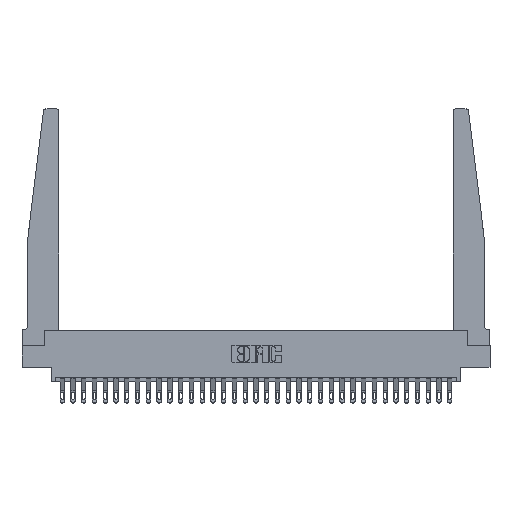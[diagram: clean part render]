
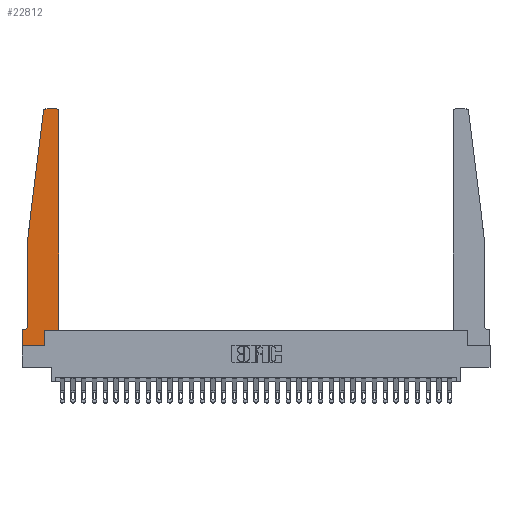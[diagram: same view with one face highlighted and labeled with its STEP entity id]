
A CAD part, top view. The second image highlights one B-rep face of the part: STEP entity #22812.
In plain terms, the highlighted planar face has unit normal (0, 0, 1).
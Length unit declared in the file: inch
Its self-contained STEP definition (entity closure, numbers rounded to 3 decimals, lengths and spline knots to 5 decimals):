
#106 = EDGE_CURVE ( 'NONE', #25178, #21801, #6517, .T. ) ;
#535 = EDGE_CURVE ( 'NONE', #23269, #25178, #2683, .T. ) ;
#1488 = EDGE_CURVE ( 'NONE', #19213, #11718, #28587, .T. ) ;
#2127 = CARTESIAN_POINT ( 'NONE',  ( 0.065, 0.2375, 0.37 ) ) ;
#2132 = VERTEX_POINT ( 'NONE', #7292 ) ;
#2136 = DIRECTION ( 'NONE',  ( 1., 0., 0. ) ) ;
#2334 = LINE ( 'NONE', #12359, #7658 ) ;
#2683 = LINE ( 'NONE', #5020, #24087 ) ;
#3017 = CARTESIAN_POINT ( 'NONE',  ( 0.2605, 0.18, 0.37 ) ) ;
#3242 = LINE ( 'NONE', #26306, #25599 ) ;
#3306 = CARTESIAN_POINT ( 'NONE',  ( 0.425, 0.18, 0.37 ) ) ;
#3314 = VERTEX_POINT ( 'NONE', #25134 ) ;
#3473 = LINE ( 'NONE', #21621, #29854 ) ;
#3608 = DIRECTION ( 'NONE',  ( 1., 0., 0. ) ) ;
#4772 = CARTESIAN_POINT ( 'NONE',  ( 0., 0., 0.37 ) ) ;
#5020 = CARTESIAN_POINT ( 'NONE',  ( 0.065, 1.25, 0.37 ) ) ;
#5546 = AXIS2_PLACEMENT_3D ( 'NONE', #10286, #24221, #7823 ) ;
#5682 = CARTESIAN_POINT ( 'NONE',  ( 0.065, 1.25, 0.37 ) ) ;
#5725 = ORIENTED_EDGE ( 'NONE', *, *, #16539, .T. ) ;
#6051 = DIRECTION ( 'NONE',  ( 0., 1., 0. ) ) ;
#6103 = DIRECTION ( 'NONE',  ( 1., 0., 0. ) ) ;
#6217 = ORIENTED_EDGE ( 'NONE', *, *, #535, .T. ) ;
#6342 = LINE ( 'NONE', #25376, #21973 ) ;
#6421 = DIRECTION ( 'NONE',  ( 0., 0., 1. ) ) ;
#6444 = ORIENTED_EDGE ( 'NONE', *, *, #16120, .T. ) ;
#6517 = CIRCLE ( 'NONE', #5546, 0.05 ) ;
#7292 = CARTESIAN_POINT ( 'NONE',  ( 0., 0., 0.37 ) ) ;
#7658 = VECTOR ( 'NONE', #21812, 39.37008 ) ;
#7823 = DIRECTION ( 'NONE',  ( -1., 0., 0. ) ) ;
#8012 = DIRECTION ( 'NONE',  ( 1., 0., 0. ) ) ;
#8994 = EDGE_CURVE ( 'NONE', #26713, #3314, #17209, .T. ) ;
#9644 = CARTESIAN_POINT ( 'NONE',  ( 0.425, 0.18, 0.37 ) ) ;
#9807 = ORIENTED_EDGE ( 'NONE', *, *, #15146, .T. ) ;
#9889 = DIRECTION ( 'NONE',  ( -1., 0., 0. ) ) ;
#10286 = CARTESIAN_POINT ( 'NONE',  ( 0.015, 0.2375, 0.37 ) ) ;
#10298 = LINE ( 'NONE', #5682, #20580 ) ;
#10486 = EDGE_CURVE ( 'NONE', #27199, #26713, #27411, .T. ) ;
#10804 = AXIS2_PLACEMENT_3D ( 'NONE', #27915, #6421, #22838 ) ;
#10860 = CARTESIAN_POINT ( 'NONE',  ( 0.395, 2.75, 0.37 ) ) ;
#11380 = LINE ( 'NONE', #4772, #18098 ) ;
#11718 = VERTEX_POINT ( 'NONE', #12896 ) ;
#11775 = DIRECTION ( 'NONE',  ( 0., 1., 0. ) ) ;
#11841 = ORIENTED_EDGE ( 'NONE', *, *, #13680, .T. ) ;
#12359 = CARTESIAN_POINT ( 'NONE',  ( 0., 0., 0.37 ) ) ;
#12484 = DIRECTION ( 'NONE',  ( 0., 0., 1. ) ) ;
#12896 = CARTESIAN_POINT ( 'NONE',  ( 0.24675, 2.72367, 0.37 ) ) ;
#13319 = CARTESIAN_POINT ( 'NONE',  ( 0.065, 1.25, 0.37 ) ) ;
#13458 = VECTOR ( 'NONE', #11775, 39.37008 ) ;
#13680 = EDGE_CURVE ( 'NONE', #11718, #23269, #10298, .T. ) ;
#14356 = CARTESIAN_POINT ( 'NONE',  ( 0.2605, 0., 0.37 ) ) ;
#15123 = ORIENTED_EDGE ( 'NONE', *, *, #8994, .T. ) ;
#15131 = CARTESIAN_POINT ( 'NONE',  ( 0., 0.1875, 0.37 ) ) ;
#15146 = EDGE_CURVE ( 'NONE', #15852, #19213, #3242, .T. ) ;
#15391 = ORIENTED_EDGE ( 'NONE', *, *, #18685, .T. ) ;
#15408 = CARTESIAN_POINT ( 'NONE',  ( 0.27653, 2.75, 0.37 ) ) ;
#15852 = VERTEX_POINT ( 'NONE', #10860 ) ;
#16120 = EDGE_CURVE ( 'NONE', #28943, #27199, #6342, .T. ) ;
#16298 = FACE_OUTER_BOUND ( 'NONE', #25149, .T. ) ;
#16539 = EDGE_CURVE ( 'NONE', #21801, #26189, #3473, .T. ) ;
#17039 = CARTESIAN_POINT ( 'NONE',  ( 0.015, 0.1875, 0.37 ) ) ;
#17209 = LINE ( 'NONE', #9644, #13458 ) ;
#17278 = CARTESIAN_POINT ( 'NONE',  ( 0.395, 2.72, 0.37 ) ) ;
#17915 = EDGE_CURVE ( 'NONE', #3314, #15852, #27969, .T. ) ;
#18098 = VECTOR ( 'NONE', #2136, 39.37008 ) ;
#18685 = EDGE_CURVE ( 'NONE', #26189, #2132, #2334, .T. ) ;
#18910 = DIRECTION ( 'NONE',  ( 0., -1., 0. ) ) ;
#19213 = VERTEX_POINT ( 'NONE', #15408 ) ;
#20157 = DIRECTION ( 'NONE',  ( -1., 0., 0. ) ) ;
#20580 = VECTOR ( 'NONE', #24856, 39.37008 ) ;
#20706 = EDGE_CURVE ( 'NONE', #2132, #28943, #11380, .T. ) ;
#20943 = ORIENTED_EDGE ( 'NONE', *, *, #20706, .T. ) ;
#21621 = CARTESIAN_POINT ( 'NONE',  ( 0.065, 0.1875, 0.37 ) ) ;
#21655 = ORIENTED_EDGE ( 'NONE', *, *, #106, .T. ) ;
#21801 = VERTEX_POINT ( 'NONE', #17039 ) ;
#21812 = DIRECTION ( 'NONE',  ( 0., -1., 0. ) ) ;
#21920 = CARTESIAN_POINT ( 'NONE',  ( 0.425, 0.18, 0.37 ) ) ;
#21973 = VECTOR ( 'NONE', #6051, 39.37008 ) ;
#22092 = DIRECTION ( 'NONE',  ( 0., 0., 1. ) ) ;
#22812 = ADVANCED_FACE ( 'NONE', ( #16298 ), #28072, .T. ) ;
#22838 = DIRECTION ( 'NONE',  ( 1., 0., 0. ) ) ;
#23269 = VERTEX_POINT ( 'NONE', #13319 ) ;
#24087 = VECTOR ( 'NONE', #18910, 39.37008 ) ;
#24124 = ORIENTED_EDGE ( 'NONE', *, *, #17915, .T. ) ;
#24221 = DIRECTION ( 'NONE',  ( 0., 0., -1. ) ) ;
#24658 = ORIENTED_EDGE ( 'NONE', *, *, #10486, .T. ) ;
#24856 = DIRECTION ( 'NONE',  ( -0.122, -0.992, 0. ) ) ;
#24993 = CARTESIAN_POINT ( 'NONE',  ( 0.27653, 2.72, 0.37 ) ) ;
#25134 = CARTESIAN_POINT ( 'NONE',  ( 0.425, 2.72, 0.37 ) ) ;
#25149 = EDGE_LOOP ( 'NONE', ( #9807, #28997, #11841, #6217, #21655, #5725, #15391, #20943, #6444, #24658, #15123, #24124 ) ) ;
#25178 = VERTEX_POINT ( 'NONE', #2127 ) ;
#25376 = CARTESIAN_POINT ( 'NONE',  ( 0.2605, 0.18, 0.37 ) ) ;
#25599 = VECTOR ( 'NONE', #9889, 39.37008 ) ;
#25622 = AXIS2_PLACEMENT_3D ( 'NONE', #24993, #12484, #6103 ) ;
#26189 = VERTEX_POINT ( 'NONE', #15131 ) ;
#26306 = CARTESIAN_POINT ( 'NONE',  ( 0.25, 2.75, 0.37 ) ) ;
#26713 = VERTEX_POINT ( 'NONE', #21920 ) ;
#27199 = VERTEX_POINT ( 'NONE', #3017 ) ;
#27411 = LINE ( 'NONE', #3306, #29855 ) ;
#27915 = CARTESIAN_POINT ( 'NONE',  ( 0., 0.1875, 0.37 ) ) ;
#27969 = CIRCLE ( 'NONE', #28471, 0.03 ) ;
#28072 = PLANE ( 'NONE',  #10804 ) ;
#28471 = AXIS2_PLACEMENT_3D ( 'NONE', #17278, #22092, #8012 ) ;
#28587 = CIRCLE ( 'NONE', #25622, 0.03 ) ;
#28943 = VERTEX_POINT ( 'NONE', #14356 ) ;
#28997 = ORIENTED_EDGE ( 'NONE', *, *, #1488, .T. ) ;
#29854 = VECTOR ( 'NONE', #20157, 39.37008 ) ;
#29855 = VECTOR ( 'NONE', #3608, 39.37008 ) ;
